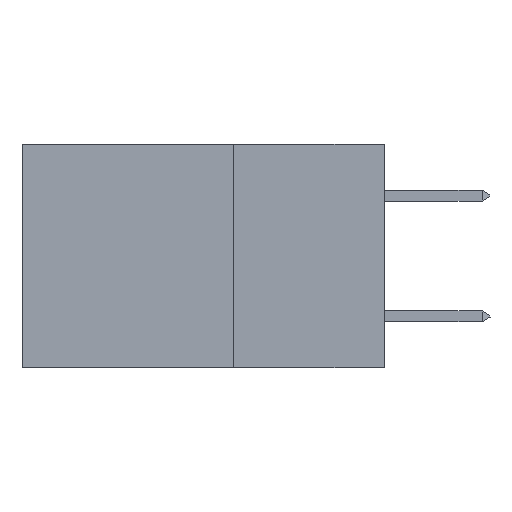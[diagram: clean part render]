
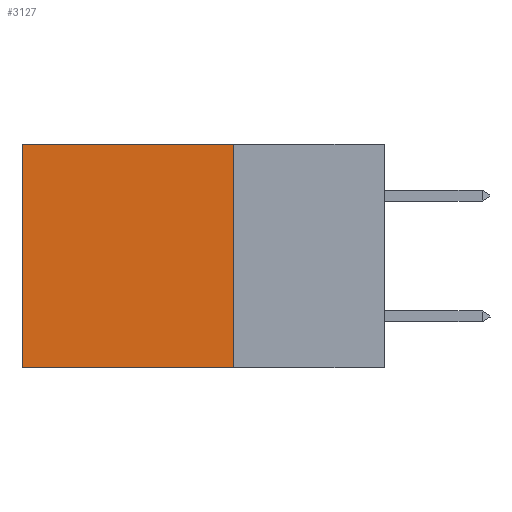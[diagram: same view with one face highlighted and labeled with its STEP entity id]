
A CAD part, left-side view. The second image highlights one B-rep face of the part: STEP entity #3127.
In plain terms, the highlighted planar face has unit normal (-1, 0, 0).
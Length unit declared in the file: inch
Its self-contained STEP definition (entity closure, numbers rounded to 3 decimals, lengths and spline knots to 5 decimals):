
#1949 = ORIENTED_EDGE ( 'NONE', *, *, #4875, .F. ) ;
#2098 = CARTESIAN_POINT ( 'NONE',  ( 0.2875, 0.6, -0.37 ) ) ;
#2389 = VECTOR ( 'NONE', #11957, 39.37008 ) ;
#3103 = EDGE_LOOP ( 'NONE', ( #10568, #12033, #1949, #17964 ) ) ;
#3127 = ADVANCED_FACE ( 'NONE', ( #16579 ), #3498, .F. ) ;
#3498 = PLANE ( 'NONE',  #16343 ) ;
#3576 = CARTESIAN_POINT ( 'NONE',  ( 0.2875, 0.25, 0. ) ) ;
#3904 = LINE ( 'NONE', #10540, #2389 ) ;
#4344 = CARTESIAN_POINT ( 'NONE',  ( 0.2875, 0.25, 0. ) ) ;
#4875 = EDGE_CURVE ( 'NONE', #17955, #5078, #3904, .T. ) ;
#5078 = VERTEX_POINT ( 'NONE', #7902 ) ;
#6037 = DIRECTION ( 'NONE',  ( 0., 1., 0. ) ) ;
#6119 = LINE ( 'NONE', #3576, #7424 ) ;
#6682 = CARTESIAN_POINT ( 'NONE',  ( 0.2875, 0.6, 0. ) ) ;
#7361 = LINE ( 'NONE', #15407, #9752 ) ;
#7424 = VECTOR ( 'NONE', #17499, 39.37008 ) ;
#7902 = CARTESIAN_POINT ( 'NONE',  ( 0.2875, 0.25, -0.37 ) ) ;
#7957 = EDGE_CURVE ( 'NONE', #5078, #16932, #10040, .T. ) ;
#8089 = VECTOR ( 'NONE', #6037, 39.37008 ) ;
#9752 = VECTOR ( 'NONE', #14021, 39.37008 ) ;
#10040 = LINE ( 'NONE', #14525, #8089 ) ;
#10489 = CARTESIAN_POINT ( 'NONE',  ( 0.2875, 0.25, 0. ) ) ;
#10540 = CARTESIAN_POINT ( 'NONE',  ( 0.2875, 0.25, 0. ) ) ;
#10568 = ORIENTED_EDGE ( 'NONE', *, *, #14406, .T. ) ;
#11957 = DIRECTION ( 'NONE',  ( 0., 0., -1. ) ) ;
#12033 = ORIENTED_EDGE ( 'NONE', *, *, #7957, .F. ) ;
#12135 = VERTEX_POINT ( 'NONE', #6682 ) ;
#12714 = EDGE_CURVE ( 'NONE', #17955, #12135, #6119, .T. ) ;
#13254 = DIRECTION ( 'NONE',  ( 1., 0., 0. ) ) ;
#14021 = DIRECTION ( 'NONE',  ( 0., 0., -1. ) ) ;
#14406 = EDGE_CURVE ( 'NONE', #12135, #16932, #7361, .T. ) ;
#14525 = CARTESIAN_POINT ( 'NONE',  ( 0.2875, 0.25, -0.37 ) ) ;
#14660 = DIRECTION ( 'NONE',  ( 0., 0., -1. ) ) ;
#15407 = CARTESIAN_POINT ( 'NONE',  ( 0.2875, 0.6, 0. ) ) ;
#16343 = AXIS2_PLACEMENT_3D ( 'NONE', #10489, #13254, #14660 ) ;
#16579 = FACE_OUTER_BOUND ( 'NONE', #3103, .T. ) ;
#16932 = VERTEX_POINT ( 'NONE', #2098 ) ;
#17499 = DIRECTION ( 'NONE',  ( 0., 1., 0. ) ) ;
#17955 = VERTEX_POINT ( 'NONE', #4344 ) ;
#17964 = ORIENTED_EDGE ( 'NONE', *, *, #12714, .T. ) ;
